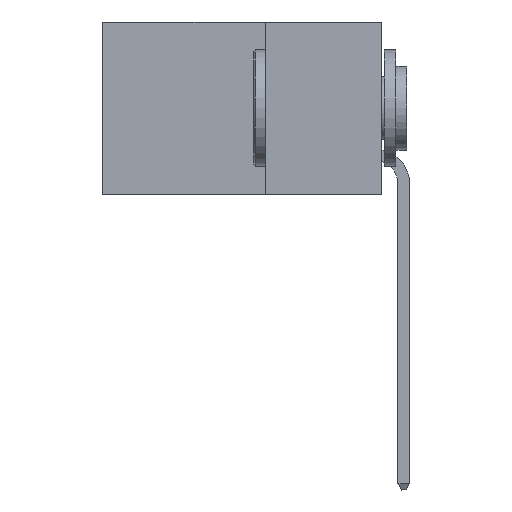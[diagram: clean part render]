
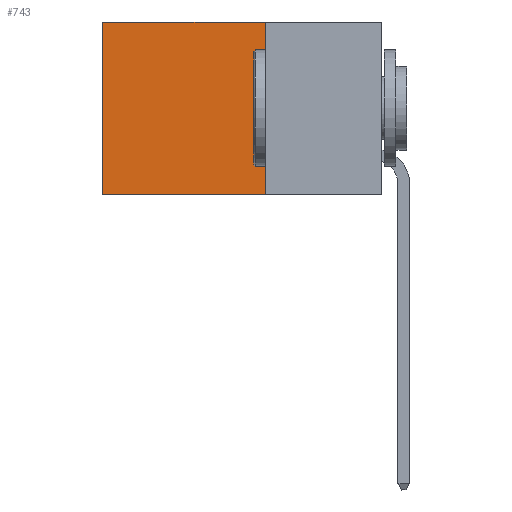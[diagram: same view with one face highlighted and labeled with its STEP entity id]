
A CAD part, left-side view. The second image highlights one B-rep face of the part: STEP entity #743.
In plain terms, the highlighted planar face has unit normal (-1, 0, 0).
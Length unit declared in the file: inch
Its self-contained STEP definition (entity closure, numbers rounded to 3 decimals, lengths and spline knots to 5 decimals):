
#14 = VERTEX_POINT ( 'NONE', #3563 ) ;
#743 = ADVANCED_FACE ( 'NONE', ( #5309 ), #10244, .F. ) ;
#819 = DIRECTION ( 'NONE',  ( 0., 0., -1. ) ) ;
#1001 = CARTESIAN_POINT ( 'NONE',  ( 0.2875, 0.25, 0. ) ) ;
#2127 = DIRECTION ( 'NONE',  ( 0., 1., 0. ) ) ;
#2522 = LINE ( 'NONE', #1001, #3545 ) ;
#2999 = VERTEX_POINT ( 'NONE', #9776 ) ;
#3292 = EDGE_CURVE ( 'NONE', #14, #11915, #2522, .T. ) ;
#3545 = VECTOR ( 'NONE', #8314, 39.37008 ) ;
#3563 = CARTESIAN_POINT ( 'NONE',  ( 0.2875, 0.25, 0. ) ) ;
#3851 = CARTESIAN_POINT ( 'NONE',  ( 0.2875, 0.25, 0. ) ) ;
#4416 = DIRECTION ( 'NONE',  ( 0., 0., -1. ) ) ;
#4591 = AXIS2_PLACEMENT_3D ( 'NONE', #3851, #5808, #12390 ) ;
#4920 = VECTOR ( 'NONE', #4416, 39.37008 ) ;
#5309 = FACE_OUTER_BOUND ( 'NONE', #6075, .T. ) ;
#5454 = ORIENTED_EDGE ( 'NONE', *, *, #8578, .T. ) ;
#5808 = DIRECTION ( 'NONE',  ( 1., 0., 0. ) ) ;
#6075 = EDGE_LOOP ( 'NONE', ( #5454, #12380, #10011, #7513 ) ) ;
#7513 = ORIENTED_EDGE ( 'NONE', *, *, #3292, .T. ) ;
#7641 = VERTEX_POINT ( 'NONE', #8949 ) ;
#8131 = CARTESIAN_POINT ( 'NONE',  ( 0.2875, 0.25, 0. ) ) ;
#8198 = VECTOR ( 'NONE', #2127, 39.37008 ) ;
#8256 = CARTESIAN_POINT ( 'NONE',  ( 0.2875, 0.6, 0. ) ) ;
#8277 = LINE ( 'NONE', #8256, #4920 ) ;
#8314 = DIRECTION ( 'NONE',  ( 0., 1., 0. ) ) ;
#8402 = CARTESIAN_POINT ( 'NONE',  ( 0.2875, 0.25, -0.37 ) ) ;
#8578 = EDGE_CURVE ( 'NONE', #11915, #2999, #8277, .T. ) ;
#8949 = CARTESIAN_POINT ( 'NONE',  ( 0.2875, 0.25, -0.37 ) ) ;
#9776 = CARTESIAN_POINT ( 'NONE',  ( 0.2875, 0.6, -0.37 ) ) ;
#9834 = VECTOR ( 'NONE', #819, 39.37008 ) ;
#10011 = ORIENTED_EDGE ( 'NONE', *, *, #10470, .F. ) ;
#10038 = CARTESIAN_POINT ( 'NONE',  ( 0.2875, 0.6, 0. ) ) ;
#10179 = LINE ( 'NONE', #8131, #9834 ) ;
#10244 = PLANE ( 'NONE',  #4591 ) ;
#10470 = EDGE_CURVE ( 'NONE', #14, #7641, #10179, .T. ) ;
#11915 = VERTEX_POINT ( 'NONE', #10038 ) ;
#12292 = EDGE_CURVE ( 'NONE', #7641, #2999, #13200, .T. ) ;
#12380 = ORIENTED_EDGE ( 'NONE', *, *, #12292, .F. ) ;
#12390 = DIRECTION ( 'NONE',  ( 0., 0., -1. ) ) ;
#13200 = LINE ( 'NONE', #8402, #8198 ) ;
